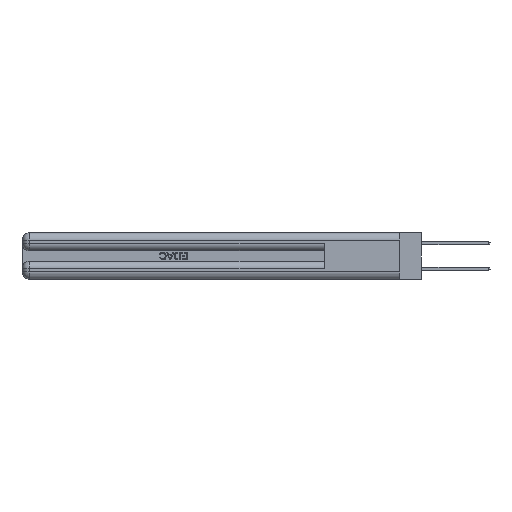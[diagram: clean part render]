
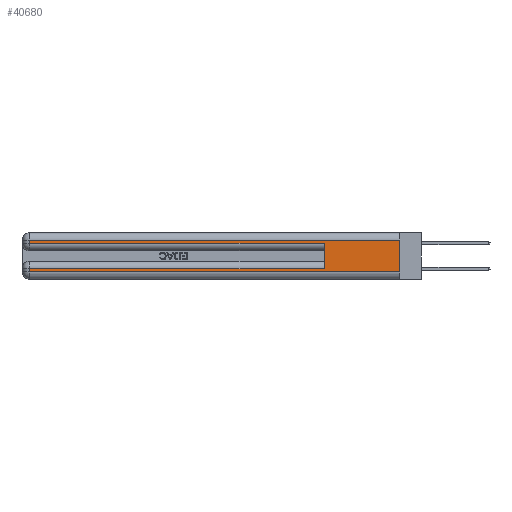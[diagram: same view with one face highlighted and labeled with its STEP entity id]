
A CAD part, left-side view. The second image highlights one B-rep face of the part: STEP entity #40680.
In plain terms, the highlighted planar face has unit normal (-1, 0, 0).
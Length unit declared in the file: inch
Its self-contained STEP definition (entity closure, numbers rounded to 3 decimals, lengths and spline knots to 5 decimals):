
#2169 = DIRECTION ( 'NONE',  ( 0., 0., -1. ) ) ;
#2519 = DIRECTION ( 'NONE',  ( 0., -1., 0. ) ) ;
#3101 = ORIENTED_EDGE ( 'NONE', *, *, #38516, .F. ) ;
#3362 = VECTOR ( 'NONE', #2169, 39.37008 ) ;
#3431 = LINE ( 'NONE', #40808, #40576 ) ;
#4541 = ORIENTED_EDGE ( 'NONE', *, *, #21599, .F. ) ;
#4820 = CARTESIAN_POINT ( 'NONE',  ( 0., 2.94, 0.37 ) ) ;
#5600 = CARTESIAN_POINT ( 'NONE',  ( 0., 2.94, 0.31 ) ) ;
#6385 = VECTOR ( 'NONE', #20560, 39.37008 ) ;
#6699 = LINE ( 'NONE', #39935, #43835 ) ;
#7339 = CARTESIAN_POINT ( 'NONE',  ( 0., 2.94, 0.06 ) ) ;
#8760 = ORIENTED_EDGE ( 'NONE', *, *, #21139, .T. ) ;
#9535 = ORIENTED_EDGE ( 'NONE', *, *, #11796, .T. ) ;
#9819 = LINE ( 'NONE', #46956, #27243 ) ;
#11796 = EDGE_CURVE ( 'NONE', #40587, #24274, #13884, .T. ) ;
#11984 = EDGE_CURVE ( 'NONE', #43743, #36887, #33019, .T. ) ;
#13884 = LINE ( 'NONE', #4820, #22574 ) ;
#14873 = DIRECTION ( 'NONE',  ( 0., -1., 0. ) ) ;
#16561 = LINE ( 'NONE', #16955, #44973 ) ;
#16835 = CARTESIAN_POINT ( 'NONE',  ( 0., 0., 0.37 ) ) ;
#16955 = CARTESIAN_POINT ( 'NONE',  ( 0., 0., 0.085 ) ) ;
#17114 = DIRECTION ( 'NONE',  ( 0., 0., -1. ) ) ;
#18378 = CARTESIAN_POINT ( 'NONE',  ( 0., 0.6, 0.285 ) ) ;
#20560 = DIRECTION ( 'NONE',  ( 0., 0., -1. ) ) ;
#21139 = EDGE_CURVE ( 'NONE', #37837, #40587, #43585, .T. ) ;
#21461 = DIRECTION ( 'NONE',  ( 0., 0., 1. ) ) ;
#21599 = EDGE_CURVE ( 'NONE', #37837, #43325, #44674, .T. ) ;
#21910 = EDGE_CURVE ( 'NONE', #24274, #30948, #3431, .T. ) ;
#22574 = VECTOR ( 'NONE', #27035, 39.37008 ) ;
#23696 = CARTESIAN_POINT ( 'NONE',  ( 0., 0., 0.31 ) ) ;
#23763 = CARTESIAN_POINT ( 'NONE',  ( 0., 0., 0.06 ) ) ;
#24274 = VERTEX_POINT ( 'NONE', #25069 ) ;
#24276 = CARTESIAN_POINT ( 'NONE',  ( 0., 2.94, 0.37 ) ) ;
#25069 = CARTESIAN_POINT ( 'NONE',  ( 0., 2.94, 0.285 ) ) ;
#26338 = ORIENTED_EDGE ( 'NONE', *, *, #43443, .T. ) ;
#27035 = DIRECTION ( 'NONE',  ( 0., 0., -1. ) ) ;
#27243 = VECTOR ( 'NONE', #2519, 39.37008 ) ;
#27985 = DIRECTION ( 'NONE',  ( 0., 1., 0. ) ) ;
#29087 = ORIENTED_EDGE ( 'NONE', *, *, #21910, .T. ) ;
#30948 = VERTEX_POINT ( 'NONE', #18378 ) ;
#31902 = PLANE ( 'NONE',  #46293 ) ;
#32076 = ORIENTED_EDGE ( 'NONE', *, *, #11984, .T. ) ;
#32313 = CARTESIAN_POINT ( 'NONE',  ( 0., 0.6, 0.085 ) ) ;
#32510 = ORIENTED_EDGE ( 'NONE', *, *, #40165, .T. ) ;
#33019 = LINE ( 'NONE', #24276, #3362 ) ;
#33249 = VERTEX_POINT ( 'NONE', #32313 ) ;
#34851 = VECTOR ( 'NONE', #45868, 39.37008 ) ;
#35616 = CARTESIAN_POINT ( 'NONE',  ( 0., 0., 0.37 ) ) ;
#36887 = VERTEX_POINT ( 'NONE', #7339 ) ;
#37079 = FACE_OUTER_BOUND ( 'NONE', #47903, .T. ) ;
#37837 = VERTEX_POINT ( 'NONE', #42752 ) ;
#38516 = EDGE_CURVE ( 'NONE', #33249, #30948, #6699, .T. ) ;
#39322 = DIRECTION ( 'NONE',  ( 1., 0., 0. ) ) ;
#39935 = CARTESIAN_POINT ( 'NONE',  ( 0., 0.6, 0.145 ) ) ;
#40165 = EDGE_CURVE ( 'NONE', #36887, #43325, #9819, .T. ) ;
#40576 = VECTOR ( 'NONE', #14873, 39.37008 ) ;
#40587 = VERTEX_POINT ( 'NONE', #5600 ) ;
#40680 = ADVANCED_FACE ( 'NONE', ( #37079 ), #31902, .F. ) ;
#40755 = CARTESIAN_POINT ( 'NONE',  ( 0., 2.94, 0.085 ) ) ;
#40808 = CARTESIAN_POINT ( 'NONE',  ( 0., 0., 0.285 ) ) ;
#42752 = CARTESIAN_POINT ( 'NONE',  ( 0., 0., 0.31 ) ) ;
#43325 = VERTEX_POINT ( 'NONE', #23763 ) ;
#43443 = EDGE_CURVE ( 'NONE', #33249, #43743, #16561, .T. ) ;
#43585 = LINE ( 'NONE', #23696, #34851 ) ;
#43743 = VERTEX_POINT ( 'NONE', #40755 ) ;
#43835 = VECTOR ( 'NONE', #21461, 39.37008 ) ;
#44674 = LINE ( 'NONE', #16835, #6385 ) ;
#44973 = VECTOR ( 'NONE', #27985, 39.37008 ) ;
#45868 = DIRECTION ( 'NONE',  ( 0., 1., 0. ) ) ;
#46293 = AXIS2_PLACEMENT_3D ( 'NONE', #35616, #39322, #17114 ) ;
#46956 = CARTESIAN_POINT ( 'NONE',  ( 0., 0., 0.06 ) ) ;
#47903 = EDGE_LOOP ( 'NONE', ( #4541, #8760, #9535, #29087, #3101, #26338, #32076, #32510 ) ) ;
